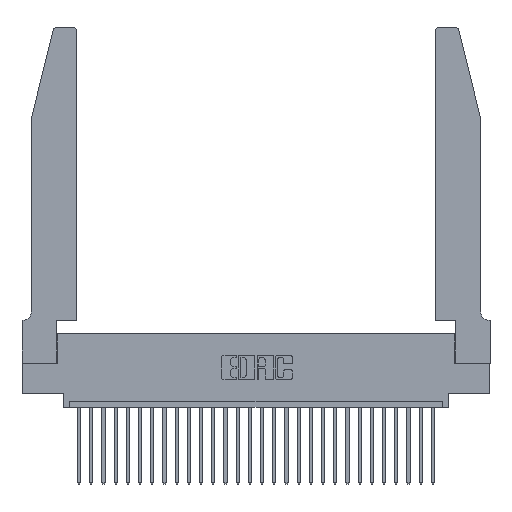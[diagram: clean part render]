
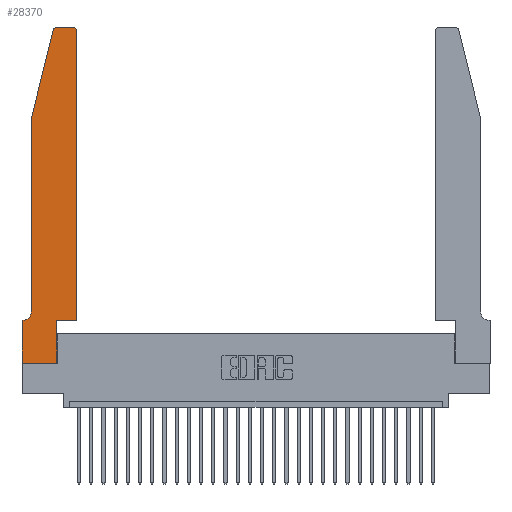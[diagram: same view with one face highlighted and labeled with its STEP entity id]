
A CAD part, top view. The second image highlights one B-rep face of the part: STEP entity #28370.
In plain terms, the highlighted planar face has unit normal (0, 0, 1).
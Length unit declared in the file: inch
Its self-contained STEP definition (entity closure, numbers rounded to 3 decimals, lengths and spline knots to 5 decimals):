
#74 = AXIS2_PLACEMENT_3D ( 'NONE', #20674, #27745, #22943 ) ;
#228 = EDGE_CURVE ( 'NONE', #20843, #23194, #17530, .T. ) ;
#351 = CARTESIAN_POINT ( 'NONE',  ( 0.0755, 2., 0.37 ) ) ;
#398 = EDGE_CURVE ( 'NONE', #17954, #23639, #4498, .T. ) ;
#669 = DIRECTION ( 'NONE',  ( 0., 0., 1. ) ) ;
#1599 = EDGE_CURVE ( 'NONE', #17784, #17954, #14305, .T. ) ;
#1974 = CIRCLE ( 'NONE', #16494, 0.03 ) ;
#2201 = CARTESIAN_POINT ( 'NONE',  ( 0.284, 2.75, 0.37 ) ) ;
#2262 = VERTEX_POINT ( 'NONE', #3339 ) ;
#2363 = VECTOR ( 'NONE', #5900, 39.37008 ) ;
#2723 = VERTEX_POINT ( 'NONE', #19759 ) ;
#2903 = CARTESIAN_POINT ( 'NONE',  ( 0.4505, 2.72, 0.37 ) ) ;
#3162 = VERTEX_POINT ( 'NONE', #2201 ) ;
#3339 = CARTESIAN_POINT ( 'NONE',  ( 0., 0.35, 0.37 ) ) ;
#3616 = DIRECTION ( 'NONE',  ( 0., 0., 1. ) ) ;
#3661 = ORIENTED_EDGE ( 'NONE', *, *, #228, .T. ) ;
#4478 = ORIENTED_EDGE ( 'NONE', *, *, #398, .T. ) ;
#4498 = LINE ( 'NONE', #21317, #12600 ) ;
#5805 = CARTESIAN_POINT ( 'NONE',  ( 0.2865, 0.35, 0.37 ) ) ;
#5900 = DIRECTION ( 'NONE',  ( 0., 1., 0. ) ) ;
#6229 = ORIENTED_EDGE ( 'NONE', *, *, #17128, .T. ) ;
#6603 = LINE ( 'NONE', #10702, #17901 ) ;
#7096 = CARTESIAN_POINT ( 'NONE',  ( 0.4205, 2.75, 0.37 ) ) ;
#7406 = VECTOR ( 'NONE', #28046, 39.37008 ) ;
#7647 = VERTEX_POINT ( 'NONE', #19325 ) ;
#9075 = DIRECTION ( 'NONE',  ( -0.239, -0.971, 0. ) ) ;
#9537 = LINE ( 'NONE', #11709, #7406 ) ;
#9867 = CARTESIAN_POINT ( 'NONE',  ( 0.2865, 0., 0.37 ) ) ;
#10414 = LINE ( 'NONE', #23814, #26957 ) ;
#10501 = DIRECTION ( 'NONE',  ( -1., 0., 0. ) ) ;
#10649 = DIRECTION ( 'NONE',  ( -1., 0., 0. ) ) ;
#10702 = CARTESIAN_POINT ( 'NONE',  ( 0., 0., 0.37 ) ) ;
#10991 = CIRCLE ( 'NONE', #18767, 0.03 ) ;
#11355 = CARTESIAN_POINT ( 'NONE',  ( 0.0755, 2., 0.37 ) ) ;
#11709 = CARTESIAN_POINT ( 'NONE',  ( 0.0755, 2., 0.37 ) ) ;
#11942 = ORIENTED_EDGE ( 'NONE', *, *, #18298, .T. ) ;
#12600 = VECTOR ( 'NONE', #27897, 39.37008 ) ;
#12826 = CARTESIAN_POINT ( 'NONE',  ( 0.25487, 2.72718, 0.37 ) ) ;
#12916 = EDGE_CURVE ( 'NONE', #2262, #26332, #24484, .T. ) ;
#13184 = VERTEX_POINT ( 'NONE', #2903 ) ;
#13270 = EDGE_CURVE ( 'NONE', #13184, #26349, #1974, .T. ) ;
#13401 = CARTESIAN_POINT ( 'NONE',  ( 0.2865, 0.35, 0.37 ) ) ;
#14143 = EDGE_CURVE ( 'NONE', #3162, #20843, #10991, .T. ) ;
#14305 = LINE ( 'NONE', #5805, #2363 ) ;
#14442 = CARTESIAN_POINT ( 'NONE',  ( 0.4205, 2.72, 0.37 ) ) ;
#14523 = PLANE ( 'NONE',  #20978 ) ;
#14668 = DIRECTION ( 'NONE',  ( 0., 0., 1. ) ) ;
#14767 = CARTESIAN_POINT ( 'NONE',  ( 0.284, 2.72, 0.37 ) ) ;
#14941 = CIRCLE ( 'NONE', #74, 0.07 ) ;
#15104 = LINE ( 'NONE', #28782, #20031 ) ;
#15305 = DIRECTION ( 'NONE',  ( 0., 1., 0. ) ) ;
#15763 = ORIENTED_EDGE ( 'NONE', *, *, #27011, .T. ) ;
#16494 = AXIS2_PLACEMENT_3D ( 'NONE', #14442, #3616, #19232 ) ;
#17128 = EDGE_CURVE ( 'NONE', #26332, #17784, #6603, .T. ) ;
#17148 = EDGE_CURVE ( 'NONE', #23639, #13184, #15104, .T. ) ;
#17530 = LINE ( 'NONE', #11355, #25635 ) ;
#17632 = CARTESIAN_POINT ( 'NONE',  ( 0.4505, 0.35, 0.37 ) ) ;
#17744 = ORIENTED_EDGE ( 'NONE', *, *, #14143, .T. ) ;
#17784 = VERTEX_POINT ( 'NONE', #9867 ) ;
#17901 = VECTOR ( 'NONE', #20499, 39.37008 ) ;
#17954 = VERTEX_POINT ( 'NONE', #13401 ) ;
#18298 = EDGE_CURVE ( 'NONE', #23194, #2723, #9537, .T. ) ;
#18699 = ORIENTED_EDGE ( 'NONE', *, *, #13270, .T. ) ;
#18767 = AXIS2_PLACEMENT_3D ( 'NONE', #14767, #14668, #23913 ) ;
#19232 = DIRECTION ( 'NONE',  ( 1., 0., 0. ) ) ;
#19325 = CARTESIAN_POINT ( 'NONE',  ( 0.0055, 0.35, 0.37 ) ) ;
#19535 = VECTOR ( 'NONE', #10649, 39.37008 ) ;
#19572 = DIRECTION ( 'NONE',  ( 0., -1., 0. ) ) ;
#19759 = CARTESIAN_POINT ( 'NONE',  ( 0.0755, 0.42, 0.37 ) ) ;
#20031 = VECTOR ( 'NONE', #15305, 39.37008 ) ;
#20499 = DIRECTION ( 'NONE',  ( 1., 0., 0. ) ) ;
#20674 = CARTESIAN_POINT ( 'NONE',  ( 0.0055, 0.42, 0.37 ) ) ;
#20843 = VERTEX_POINT ( 'NONE', #12826 ) ;
#20978 = AXIS2_PLACEMENT_3D ( 'NONE', #27775, #669, #23570 ) ;
#21317 = CARTESIAN_POINT ( 'NONE',  ( 0.4505, 0.35, 0.37 ) ) ;
#21473 = EDGE_LOOP ( 'NONE', ( #24395, #17744, #3661, #11942, #15763, #28635, #25797, #6229, #23181, #4478, #28450, #18699 ) ) ;
#21896 = CARTESIAN_POINT ( 'NONE',  ( 0.2605, 2.75, 0.37 ) ) ;
#22943 = DIRECTION ( 'NONE',  ( -1., 0., 0. ) ) ;
#23181 = ORIENTED_EDGE ( 'NONE', *, *, #1599, .T. ) ;
#23194 = VERTEX_POINT ( 'NONE', #351 ) ;
#23570 = DIRECTION ( 'NONE',  ( 1., 0., 0. ) ) ;
#23639 = VERTEX_POINT ( 'NONE', #17632 ) ;
#23814 = CARTESIAN_POINT ( 'NONE',  ( 0.0755, 0.35, 0.37 ) ) ;
#23913 = DIRECTION ( 'NONE',  ( 1., 0., 0. ) ) ;
#24395 = ORIENTED_EDGE ( 'NONE', *, *, #26834, .T. ) ;
#24484 = LINE ( 'NONE', #28907, #25493 ) ;
#24737 = CARTESIAN_POINT ( 'NONE',  ( 0., 0., 0.37 ) ) ;
#25011 = FACE_OUTER_BOUND ( 'NONE', #21473, .T. ) ;
#25493 = VECTOR ( 'NONE', #19572, 39.37008 ) ;
#25635 = VECTOR ( 'NONE', #9075, 39.37008 ) ;
#25761 = EDGE_CURVE ( 'NONE', #7647, #2262, #10414, .T. ) ;
#25797 = ORIENTED_EDGE ( 'NONE', *, *, #12916, .T. ) ;
#25834 = LINE ( 'NONE', #21896, #19535 ) ;
#26332 = VERTEX_POINT ( 'NONE', #24737 ) ;
#26349 = VERTEX_POINT ( 'NONE', #7096 ) ;
#26834 = EDGE_CURVE ( 'NONE', #26349, #3162, #25834, .T. ) ;
#26957 = VECTOR ( 'NONE', #10501, 39.37008 ) ;
#27011 = EDGE_CURVE ( 'NONE', #2723, #7647, #14941, .T. ) ;
#27745 = DIRECTION ( 'NONE',  ( 0., 0., -1. ) ) ;
#27775 = CARTESIAN_POINT ( 'NONE',  ( 0., 0.35, 0.37 ) ) ;
#27897 = DIRECTION ( 'NONE',  ( 1., 0., 0. ) ) ;
#28046 = DIRECTION ( 'NONE',  ( 0., -1., 0. ) ) ;
#28370 = ADVANCED_FACE ( 'NONE', ( #25011 ), #14523, .T. ) ;
#28450 = ORIENTED_EDGE ( 'NONE', *, *, #17148, .T. ) ;
#28635 = ORIENTED_EDGE ( 'NONE', *, *, #25761, .T. ) ;
#28782 = CARTESIAN_POINT ( 'NONE',  ( 0.4505, 0.35, 0.37 ) ) ;
#28907 = CARTESIAN_POINT ( 'NONE',  ( 0., 0., 0.37 ) ) ;
